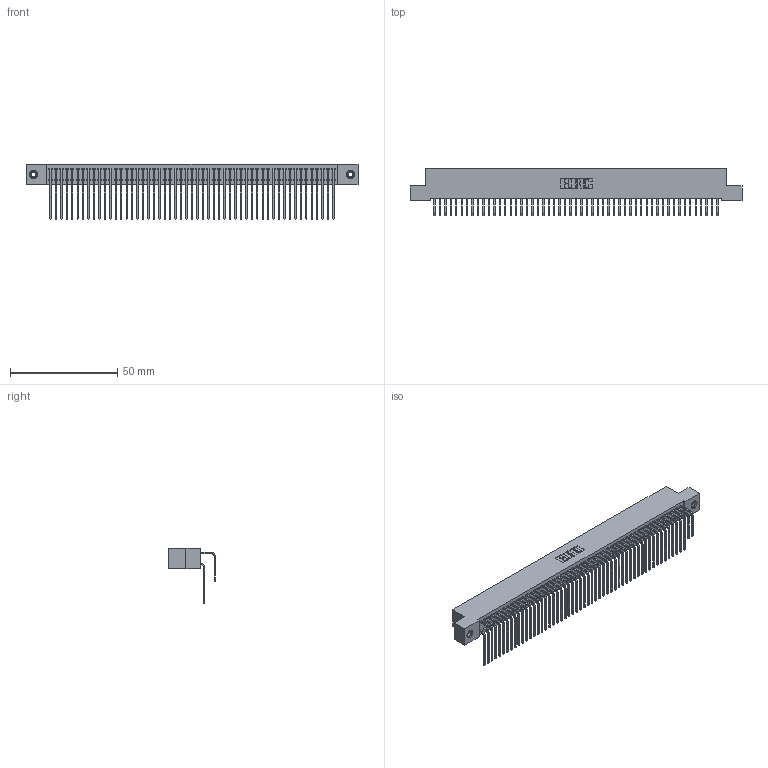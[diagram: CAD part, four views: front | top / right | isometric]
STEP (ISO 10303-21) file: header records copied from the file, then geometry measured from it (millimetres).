
FILE_DESCRIPTION (( 'STEP AP203' ), '1' );
FILE_NAME ('342-106-558-208.STEP', '2019-10-04T19:27:06', ( '' ), ( '' ), 'SwSTEP 2.0', 'SolidWorks 2016', '' );
FILE_SCHEMA (( 'CONFIG_CONTROL_DESIGN' ));
Length unit declared in the file: inch
Products named in the file (5): 345-292-001_558 Tail - 2; 345-250-001_345-250-003-102; 342-106-558-208; 342 Part_TI; 345-292-001_558 559 Tail - 1
Assembly tree (109 placements, depth 2):
  342-106-558-208
    342 Part_TI
    345-292-001_558 559 Tail - 1  x53
    345-292-001_558 Tail - 2  x53
    345-250-001_345-250-003-102  x2
Bounding box: 154.94 x 21.91 x 25.78 mm (x, y, z)
Volume: 14579.2 mm3; surface area: 26778.8 mm2
Topology: 109 solids, 109 shells, 5894 faces, 17501 edges, 11518 vertices
Faces by surface type: plane 4126, cylinder 1752, cone 12, torus 4
Entity records: 35512 total; most frequent: CARTESIAN_POINT 5904, ORIENTED_EDGE 5782, DIRECTION 5037, EDGE_CURVE 2891, VECTOR 2703, LINE 2703, VERTEX_POINT 1920, AXIS2_PLACEMENT_3D 1167
